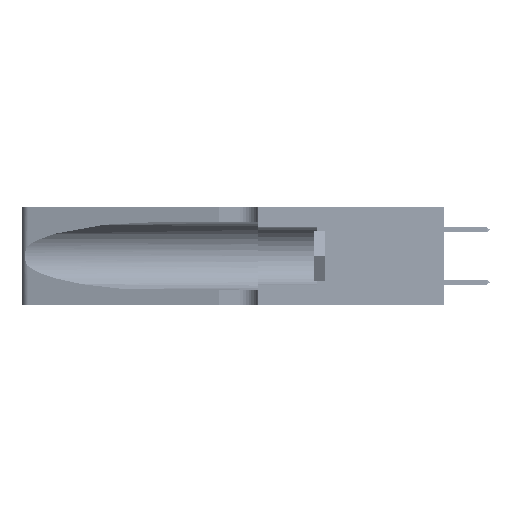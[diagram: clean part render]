
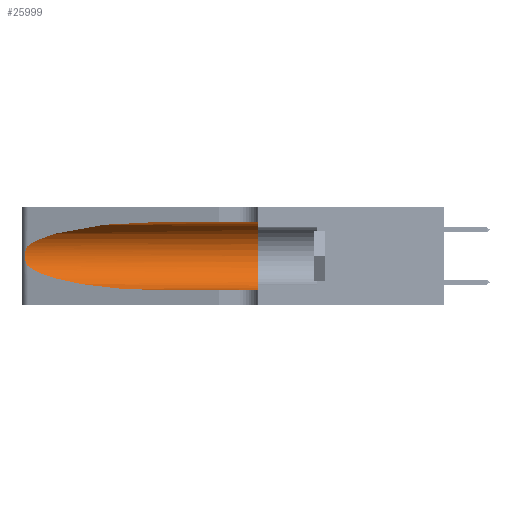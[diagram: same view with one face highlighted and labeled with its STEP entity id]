
A CAD part, left-side view. The second image highlights one B-rep face of the part: STEP entity #25999.
In plain terms, the highlighted cylindrical face has radius 3.308 mm (diameter 6.617 mm), a partial arc.
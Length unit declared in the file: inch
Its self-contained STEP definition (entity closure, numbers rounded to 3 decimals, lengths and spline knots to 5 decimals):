
#1261 = CARTESIAN_POINT ( 'NONE',  ( 0.25555, 1.22994, 0.2215 ) ) ;
#1428 = CARTESIAN_POINT ( 'NONE',  ( 0.26075, 1.23896, 0.19203 ) ) ;
#1810 = CARTESIAN_POINT ( 'NONE',  ( 0.1305, 0.35, 0.31525 ) ) ;
#4181 = CARTESIAN_POINT ( 'NONE',  ( 0.1305, 0.72297, 0.05475 ) ) ;
#4944 = CARTESIAN_POINT ( 'NONE',  ( 0.25487, 1.22718, 0.14631 ) ) ;
#5308 = CARTESIAN_POINT ( 'NONE',  ( 0.1305, 0.35, 0.185 ) ) ;
#5553 = ORIENTED_EDGE ( 'NONE', *, *, #24886, .F. ) ;
#5559 = CARTESIAN_POINT ( 'NONE',  ( 0.26017, 1.23833, 0.17102 ) ) ;
#5862 = VERTEX_POINT ( 'NONE', #4181 ) ;
#6547 = DIRECTION ( 'NONE',  ( 0., -1., 0. ) ) ;
#7918 = CARTESIAN_POINT ( 'NONE',  ( 0.25487, 1.22718, 0.22369 ) ) ;
#8200 = CARTESIAN_POINT ( 'NONE',  ( 0.25487, 1.22718, 0.14631 ) ) ;
#9419 = DIRECTION ( 'NONE',  ( 0., 0., 1. ) ) ;
#9663 = CARTESIAN_POINT ( 'NONE',  ( 0.25789, 1.23486, 0.15765 ) ) ;
#10566 = VECTOR ( 'NONE', #6547, 39.37008 ) ;
#10699 = EDGE_CURVE ( 'NONE', #33844, #5862, #39133, .T. ) ;
#11885 = LINE ( 'NONE', #43236, #10566 ) ;
#11918 = ORIENTED_EDGE ( 'NONE', *, *, #47835, .T. ) ;
#13144 = CARTESIAN_POINT ( 'NONE',  ( 0.18966, 0.96281, 0.05475 ) ) ;
#13765 = CARTESIAN_POINT ( 'NONE',  ( 0.25555, 1.22993, 0.14849 ) ) ;
#14509 = EDGE_LOOP ( 'NONE', ( #17037, #38214, #31155, #11918, #15745, #5553 ) ) ;
#14896 = CARTESIAN_POINT ( 'NONE',  ( 0.1305, 0.72297, 0.31525 ) ) ;
#15745 = ORIENTED_EDGE ( 'NONE', *, *, #42001, .F. ) ;
#16155 = B_SPLINE_CURVE_WITH_KNOTS ( 'NONE', 3,
 ( #29879, #1261, #46327, #21800, #50420, #25912, #1428, #30048, #5559, #34193, #9663, #38291, #13765, #42420 ),
 .UNSPECIFIED., .F., .F.,
 ( 4, 2, 2, 2, 2, 2, 4 ),
 ( 0., 0.00027, 0.00053, 0.00107, 0.0016, 0.00187, 0.00214 ),
 .UNSPECIFIED. ) ;
#17037 = ORIENTED_EDGE ( 'NONE', *, *, #46671, .T. ) ;
#17073 = CARTESIAN_POINT ( 'NONE',  ( 0.2373, 1.15595, 0.08982 ) ) ;
#17409 = DIRECTION ( 'NONE',  ( 0., -1., 0. ) ) ;
#17963 = VERTEX_POINT ( 'NONE', #44463 ) ;
#20027 = VERTEX_POINT ( 'NONE', #45117 ) ;
#21142 = VERTEX_POINT ( 'NONE', #14896 ) ;
#21719 =( BOUNDED_CURVE ( )  B_SPLINE_CURVE ( 3, ( #48693, #44616, #32432, #7918 ),
 .UNSPECIFIED., .F., .T. ) 
 B_SPLINE_CURVE_WITH_KNOTS ( ( 4, 4 ),
 ( 1.5708, 2.84003 ),
 .UNSPECIFIED. ) 
 CURVE ( )  GEOMETRIC_REPRESENTATION_ITEM ( )  RATIONAL_B_SPLINE_CURVE ( ( 1., 0.87, 0.87, 1. ) ) 
 REPRESENTATION_ITEM ( '' )  );
#21800 = CARTESIAN_POINT ( 'NONE',  ( 0.25787, 1.23484, 0.2124 ) ) ;
#24886 = EDGE_CURVE ( 'NONE', #21142, #29222, #25231, .T. ) ;
#25231 = LINE ( 'NONE', #50148, #34855 ) ;
#25912 = CARTESIAN_POINT ( 'NONE',  ( 0.26018, 1.23835, 0.19895 ) ) ;
#25999 = ADVANCED_FACE ( 'NONE', ( #37358 ), #26407, .F. ) ;
#26407 = CYLINDRICAL_SURFACE ( 'NONE', #44043, 0.13025 ) ;
#29222 = VERTEX_POINT ( 'NONE', #1810 ) ;
#29879 = CARTESIAN_POINT ( 'NONE',  ( 0.25487, 1.22718, 0.22369 ) ) ;
#30048 = CARTESIAN_POINT ( 'NONE',  ( 0.26075, 1.23896, 0.178 ) ) ;
#31155 = ORIENTED_EDGE ( 'NONE', *, *, #10699, .T. ) ;
#31398 = EDGE_CURVE ( 'NONE', #17963, #33844, #16155, .T. ) ;
#32432 = CARTESIAN_POINT ( 'NONE',  ( 0.2373, 1.15595, 0.28018 ) ) ;
#33844 = VERTEX_POINT ( 'NONE', #8200 ) ;
#33946 = DIRECTION ( 'NONE',  ( 0., 1., 0. ) ) ;
#34193 = CARTESIAN_POINT ( 'NONE',  ( 0.25856, 1.23593, 0.16098 ) ) ;
#34855 = VECTOR ( 'NONE', #17409, 39.37008 ) ;
#37358 = FACE_OUTER_BOUND ( 'NONE', #14509, .T. ) ;
#38214 = ORIENTED_EDGE ( 'NONE', *, *, #31398, .T. ) ;
#38291 = CARTESIAN_POINT ( 'NONE',  ( 0.25639, 1.23186, 0.15144 ) ) ;
#39133 =( BOUNDED_CURVE ( )  B_SPLINE_CURVE ( 3, ( #4944, #17073, #13144, #41782 ),
 .UNSPECIFIED., .F., .F. ) 
 B_SPLINE_CURVE_WITH_KNOTS ( ( 4, 4 ),
 ( 3.44316, 4.71239 ),
 .UNSPECIFIED. ) 
 CURVE ( )  GEOMETRIC_REPRESENTATION_ITEM ( )  RATIONAL_B_SPLINE_CURVE ( ( 1., 0.87, 0.87, 1. ) ) 
 REPRESENTATION_ITEM ( '' )  );
#41013 = AXIS2_PLACEMENT_3D ( 'NONE', #5308, #33946, #9419 ) ;
#41782 = CARTESIAN_POINT ( 'NONE',  ( 0.1305, 0.72297, 0.05475 ) ) ;
#42001 = EDGE_CURVE ( 'NONE', #29222, #20027, #42613, .T. ) ;
#42420 = CARTESIAN_POINT ( 'NONE',  ( 0.25487, 1.22718, 0.14631 ) ) ;
#42613 = CIRCLE ( 'NONE', #41013, 0.13025 ) ;
#43236 = CARTESIAN_POINT ( 'NONE',  ( 0.1305, 1.61858, 0.05475 ) ) ;
#44043 = AXIS2_PLACEMENT_3D ( 'NONE', #52535, #44547, #48623 ) ;
#44463 = CARTESIAN_POINT ( 'NONE',  ( 0.25487, 1.22718, 0.22369 ) ) ;
#44547 = DIRECTION ( 'NONE',  ( 0., -1., 0. ) ) ;
#44616 = CARTESIAN_POINT ( 'NONE',  ( 0.18966, 0.96281, 0.31525 ) ) ;
#45117 = CARTESIAN_POINT ( 'NONE',  ( 0.1305, 0.35, 0.05475 ) ) ;
#46327 = CARTESIAN_POINT ( 'NONE',  ( 0.25639, 1.23184, 0.21858 ) ) ;
#46671 = EDGE_CURVE ( 'NONE', #21142, #17963, #21719, .T. ) ;
#47835 = EDGE_CURVE ( 'NONE', #5862, #20027, #11885, .T. ) ;
#48623 = DIRECTION ( 'NONE',  ( 0., 0., -1. ) ) ;
#48693 = CARTESIAN_POINT ( 'NONE',  ( 0.1305, 0.72297, 0.31525 ) ) ;
#50148 = CARTESIAN_POINT ( 'NONE',  ( 0.1305, 1.61858, 0.31525 ) ) ;
#50420 = CARTESIAN_POINT ( 'NONE',  ( 0.25854, 1.2359, 0.20912 ) ) ;
#52535 = CARTESIAN_POINT ( 'NONE',  ( 0.1305, 1.61858, 0.185 ) ) ;
